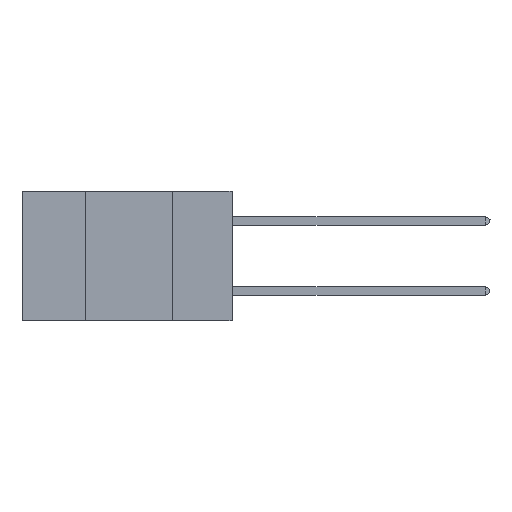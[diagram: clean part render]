
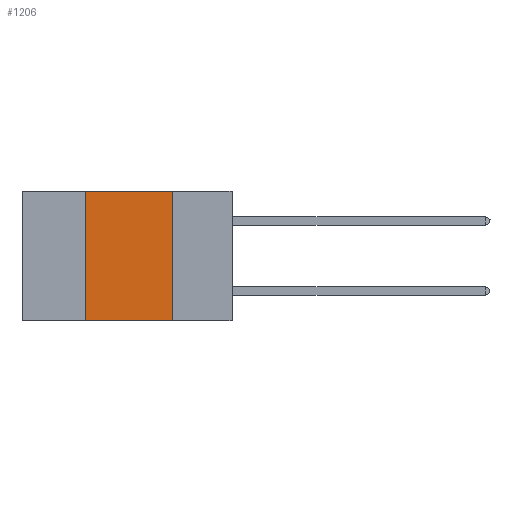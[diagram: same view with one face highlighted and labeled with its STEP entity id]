
A CAD part, left-side view. The second image highlights one B-rep face of the part: STEP entity #1206.
In plain terms, the highlighted planar face has unit normal (-1, 0, 0).
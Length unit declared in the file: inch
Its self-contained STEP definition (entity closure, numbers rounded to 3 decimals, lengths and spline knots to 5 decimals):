
#40 = DIRECTION ( 'NONE',  ( 0., -1., 0. ) ) ;
#583 = VERTEX_POINT ( 'NONE', #10658 ) ;
#672 = FACE_OUTER_BOUND ( 'NONE', #11181, .T. ) ;
#798 = ORIENTED_EDGE ( 'NONE', *, *, #1705, .F. ) ;
#977 = LINE ( 'NONE', #4308, #11288 ) ;
#1065 = AXIS2_PLACEMENT_3D ( 'NONE', #7147, #2738, #1813 ) ;
#1206 = ADVANCED_FACE ( 'NONE', ( #672 ), #4937, .F. ) ;
#1286 = CARTESIAN_POINT ( 'NONE',  ( 0., 0.17, 0. ) ) ;
#1291 = ORIENTED_EDGE ( 'NONE', *, *, #1545, .F. ) ;
#1545 = EDGE_CURVE ( 'NONE', #2720, #583, #11013, .T. ) ;
#1705 = EDGE_CURVE ( 'NONE', #9431, #13380, #12451, .T. ) ;
#1732 = CARTESIAN_POINT ( 'NONE',  ( 0., 0.42, 0. ) ) ;
#1813 = DIRECTION ( 'NONE',  ( 0., 0., -1. ) ) ;
#2049 = DIRECTION ( 'NONE',  ( 0., -1., 0. ) ) ;
#2720 = VERTEX_POINT ( 'NONE', #4169 ) ;
#2738 = DIRECTION ( 'NONE',  ( 1., 0., 0. ) ) ;
#3569 = DIRECTION ( 'NONE',  ( 0., 0., -1. ) ) ;
#3905 = EDGE_CURVE ( 'NONE', #13380, #2720, #12838, .T. ) ;
#4169 = CARTESIAN_POINT ( 'NONE',  ( 0., 0.17, 0. ) ) ;
#4308 = CARTESIAN_POINT ( 'NONE',  ( 0., 0.6, -0.37 ) ) ;
#4937 = PLANE ( 'NONE',  #1065 ) ;
#5200 = ORIENTED_EDGE ( 'NONE', *, *, #6881, .T. ) ;
#5532 = ORIENTED_EDGE ( 'NONE', *, *, #3905, .F. ) ;
#6081 = VECTOR ( 'NONE', #3569, 39.37008 ) ;
#6881 = EDGE_CURVE ( 'NONE', #9431, #583, #977, .T. ) ;
#7147 = CARTESIAN_POINT ( 'NONE',  ( 0., 0.6, 0. ) ) ;
#7296 = CARTESIAN_POINT ( 'NONE',  ( 0., 0.6, 0. ) ) ;
#9431 = VERTEX_POINT ( 'NONE', #12799 ) ;
#9909 = VECTOR ( 'NONE', #10386, 39.37008 ) ;
#10386 = DIRECTION ( 'NONE',  ( 0., 0., 1. ) ) ;
#10658 = CARTESIAN_POINT ( 'NONE',  ( 0., 0.17, -0.37 ) ) ;
#11013 = LINE ( 'NONE', #1286, #6081 ) ;
#11181 = EDGE_LOOP ( 'NONE', ( #1291, #5532, #798, #5200 ) ) ;
#11288 = VECTOR ( 'NONE', #40, 39.37008 ) ;
#12451 = LINE ( 'NONE', #13730, #9909 ) ;
#12507 = VECTOR ( 'NONE', #2049, 39.37008 ) ;
#12799 = CARTESIAN_POINT ( 'NONE',  ( 0., 0.42, -0.37 ) ) ;
#12838 = LINE ( 'NONE', #7296, #12507 ) ;
#13380 = VERTEX_POINT ( 'NONE', #1732 ) ;
#13730 = CARTESIAN_POINT ( 'NONE',  ( 0., 0.42, 0. ) ) ;
